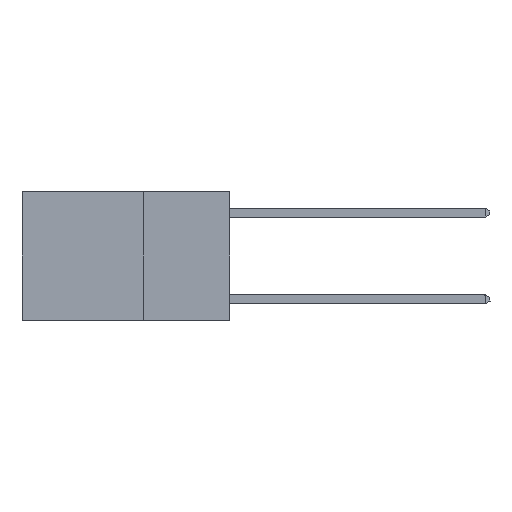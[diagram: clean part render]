
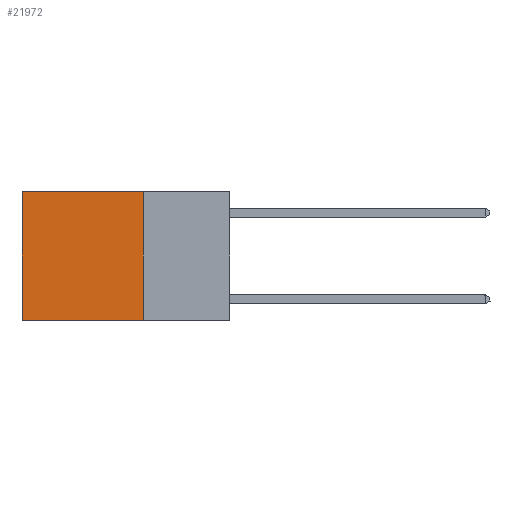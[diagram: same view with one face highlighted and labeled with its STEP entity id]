
A CAD part, left-side view. The second image highlights one B-rep face of the part: STEP entity #21972.
In plain terms, the highlighted planar face has unit normal (-1, 0, 0).
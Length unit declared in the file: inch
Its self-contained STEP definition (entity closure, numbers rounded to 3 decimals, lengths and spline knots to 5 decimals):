
#469 = CARTESIAN_POINT ( 'NONE',  ( 0.2625, 0.25, 0. ) ) ;
#1641 = EDGE_CURVE ( 'NONE', #16558, #7309, #12084, .T. ) ;
#1874 = DIRECTION ( 'NONE',  ( 0., 1., 0. ) ) ;
#2186 = CARTESIAN_POINT ( 'NONE',  ( 0.2625, 0.6, 0. ) ) ;
#2383 = DIRECTION ( 'NONE',  ( 0., 0., -1. ) ) ;
#3098 = VECTOR ( 'NONE', #11087, 39.37008 ) ;
#4063 = DIRECTION ( 'NONE',  ( 0., 0., -1. ) ) ;
#4103 = CARTESIAN_POINT ( 'NONE',  ( 0.2625, 0.6, 0. ) ) ;
#4123 = CARTESIAN_POINT ( 'NONE',  ( 0.2625, 0.25, 0. ) ) ;
#4271 = LINE ( 'NONE', #5517, #3098 ) ;
#4814 = CARTESIAN_POINT ( 'NONE',  ( 0.2625, 0.6, -0.37 ) ) ;
#5422 = EDGE_LOOP ( 'NONE', ( #23017, #12439, #11271, #7036 ) ) ;
#5517 = CARTESIAN_POINT ( 'NONE',  ( 0.2625, 0.25, -0.37 ) ) ;
#6879 = CARTESIAN_POINT ( 'NONE',  ( 0.2625, 0.25, -0.37 ) ) ;
#6881 = CARTESIAN_POINT ( 'NONE',  ( 0.2625, 0.25, 0. ) ) ;
#6962 = DIRECTION ( 'NONE',  ( 0., 0., -1. ) ) ;
#7036 = ORIENTED_EDGE ( 'NONE', *, *, #8886, .T. ) ;
#7309 = VERTEX_POINT ( 'NONE', #6879 ) ;
#7829 = VECTOR ( 'NONE', #4063, 39.37008 ) ;
#8154 = VECTOR ( 'NONE', #1874, 39.37008 ) ;
#8886 = EDGE_CURVE ( 'NONE', #16558, #17111, #21621, .T. ) ;
#9171 = VERTEX_POINT ( 'NONE', #4814 ) ;
#9548 = EDGE_CURVE ( 'NONE', #17111, #9171, #22441, .T. ) ;
#9760 = PLANE ( 'NONE',  #17782 ) ;
#11087 = DIRECTION ( 'NONE',  ( 0., 1., 0. ) ) ;
#11271 = ORIENTED_EDGE ( 'NONE', *, *, #1641, .F. ) ;
#12084 = LINE ( 'NONE', #6881, #20640 ) ;
#12439 = ORIENTED_EDGE ( 'NONE', *, *, #18280, .F. ) ;
#13442 = DIRECTION ( 'NONE',  ( 1., 0., 0. ) ) ;
#14793 = CARTESIAN_POINT ( 'NONE',  ( 0.2625, 0.25, 0. ) ) ;
#15802 = FACE_OUTER_BOUND ( 'NONE', #5422, .T. ) ;
#16558 = VERTEX_POINT ( 'NONE', #4123 ) ;
#17111 = VERTEX_POINT ( 'NONE', #4103 ) ;
#17782 = AXIS2_PLACEMENT_3D ( 'NONE', #469, #13442, #2383 ) ;
#18280 = EDGE_CURVE ( 'NONE', #7309, #9171, #4271, .T. ) ;
#20640 = VECTOR ( 'NONE', #6962, 39.37008 ) ;
#21621 = LINE ( 'NONE', #14793, #8154 ) ;
#21972 = ADVANCED_FACE ( 'NONE', ( #15802 ), #9760, .F. ) ;
#22441 = LINE ( 'NONE', #2186, #7829 ) ;
#23017 = ORIENTED_EDGE ( 'NONE', *, *, #9548, .T. ) ;
